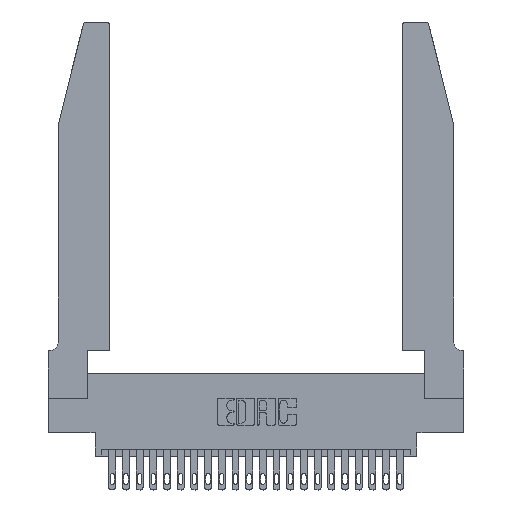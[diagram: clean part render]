
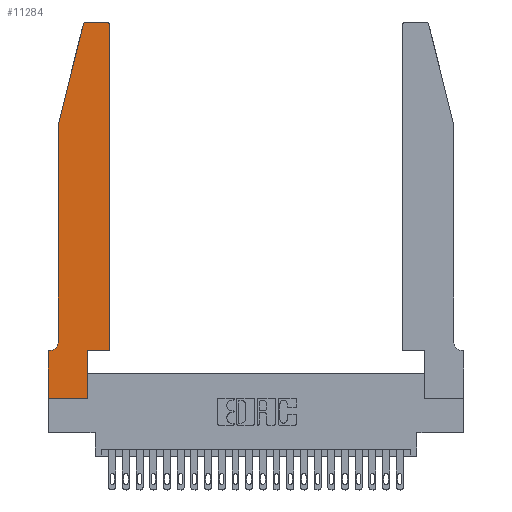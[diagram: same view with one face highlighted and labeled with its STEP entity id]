
A CAD part, top view. The second image highlights one B-rep face of the part: STEP entity #11284.
In plain terms, the highlighted planar face has unit normal (0, 0, 1).
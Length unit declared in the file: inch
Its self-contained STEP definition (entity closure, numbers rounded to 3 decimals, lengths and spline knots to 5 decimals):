
#243 = CARTESIAN_POINT ( 'NONE',  ( 0., 0., 0.37 ) ) ;
#632 = CARTESIAN_POINT ( 'NONE',  ( 0.284, 2.72, 0.37 ) ) ;
#1090 = DIRECTION ( 'NONE',  ( 0., 1., 0. ) ) ;
#1114 = AXIS2_PLACEMENT_3D ( 'NONE', #22229, #24005, #10795 ) ;
#1172 = ORIENTED_EDGE ( 'NONE', *, *, #23005, .T. ) ;
#1289 = CARTESIAN_POINT ( 'NONE',  ( 0.4505, 0.35, 0.37 ) ) ;
#1506 = CARTESIAN_POINT ( 'NONE',  ( 0.0755, 2., 0.37 ) ) ;
#1558 = EDGE_CURVE ( 'NONE', #6737, #5088, #21562, .T. ) ;
#1679 = VECTOR ( 'NONE', #21174, 39.37008 ) ;
#2625 = EDGE_CURVE ( 'NONE', #9777, #20598, #21193, .T. ) ;
#3010 = CARTESIAN_POINT ( 'NONE',  ( 0.4505, 0.35, 0.37 ) ) ;
#3607 = VERTEX_POINT ( 'NONE', #9351 ) ;
#4020 = VECTOR ( 'NONE', #17602, 39.37008 ) ;
#4476 = VERTEX_POINT ( 'NONE', #9982 ) ;
#4489 = ORIENTED_EDGE ( 'NONE', *, *, #22516, .T. ) ;
#4597 = EDGE_CURVE ( 'NONE', #6879, #9777, #5947, .T. ) ;
#5088 = VERTEX_POINT ( 'NONE', #24771 ) ;
#5301 = VECTOR ( 'NONE', #10873, 39.37008 ) ;
#5439 = VERTEX_POINT ( 'NONE', #10442 ) ;
#5543 = CARTESIAN_POINT ( 'NONE',  ( 0.2865, 0.35, 0.37 ) ) ;
#5947 = LINE ( 'NONE', #21570, #7403 ) ;
#6316 = CARTESIAN_POINT ( 'NONE',  ( 0., 0.35, 0.37 ) ) ;
#6472 = EDGE_LOOP ( 'NONE', ( #16939, #22585, #20872, #4489, #13615, #19061, #1172, #21306, #22916, #13959, #22687, #8052 ) ) ;
#6713 = LINE ( 'NONE', #8328, #7008 ) ;
#6737 = VERTEX_POINT ( 'NONE', #15553 ) ;
#6823 = VECTOR ( 'NONE', #16978, 39.37008 ) ;
#6879 = VERTEX_POINT ( 'NONE', #12028 ) ;
#7008 = VECTOR ( 'NONE', #12144, 39.37008 ) ;
#7403 = VECTOR ( 'NONE', #21819, 39.37008 ) ;
#7823 = AXIS2_PLACEMENT_3D ( 'NONE', #632, #19560, #13900 ) ;
#7963 = LINE ( 'NONE', #13411, #1679 ) ;
#7984 = DIRECTION ( 'NONE',  ( 1., 0., 0. ) ) ;
#8018 = EDGE_CURVE ( 'NONE', #11423, #15304, #6713, .T. ) ;
#8052 = ORIENTED_EDGE ( 'NONE', *, *, #22491, .T. ) ;
#8270 = CIRCLE ( 'NONE', #1114, 0.03 ) ;
#8328 = CARTESIAN_POINT ( 'NONE',  ( 0.0755, 2., 0.37 ) ) ;
#8665 = VECTOR ( 'NONE', #1090, 39.37008 ) ;
#9351 = CARTESIAN_POINT ( 'NONE',  ( 0.284, 2.75, 0.37 ) ) ;
#9777 = VERTEX_POINT ( 'NONE', #1289 ) ;
#9982 = CARTESIAN_POINT ( 'NONE',  ( 0.4205, 2.75, 0.37 ) ) ;
#10442 = CARTESIAN_POINT ( 'NONE',  ( 0., 0., 0.37 ) ) ;
#10482 = CARTESIAN_POINT ( 'NONE',  ( 0.25487, 2.72718, 0.37 ) ) ;
#10795 = DIRECTION ( 'NONE',  ( 1., 0., 0. ) ) ;
#10873 = DIRECTION ( 'NONE',  ( 0., -1., 0. ) ) ;
#11075 = VECTOR ( 'NONE', #13660, 39.37008 ) ;
#11284 = ADVANCED_FACE ( 'NONE', ( #23284 ), #14061, .T. ) ;
#11423 = VERTEX_POINT ( 'NONE', #10482 ) ;
#11638 = EDGE_CURVE ( 'NONE', #21131, #6879, #20835, .T. ) ;
#12028 = CARTESIAN_POINT ( 'NONE',  ( 0.2865, 0.35, 0.37 ) ) ;
#12144 = DIRECTION ( 'NONE',  ( -0.239, -0.971, 0. ) ) ;
#12452 = LINE ( 'NONE', #12698, #5301 ) ;
#12698 = CARTESIAN_POINT ( 'NONE',  ( 0.0755, 2., 0.37 ) ) ;
#13148 = VERTEX_POINT ( 'NONE', #19773 ) ;
#13311 = DIRECTION ( 'NONE',  ( 0., 0., -1. ) ) ;
#13411 = CARTESIAN_POINT ( 'NONE',  ( 0.0755, 0.35, 0.37 ) ) ;
#13615 = ORIENTED_EDGE ( 'NONE', *, *, #1558, .T. ) ;
#13660 = DIRECTION ( 'NONE',  ( 1., 0., 0. ) ) ;
#13900 = DIRECTION ( 'NONE',  ( 1., 0., 0. ) ) ;
#13959 = ORIENTED_EDGE ( 'NONE', *, *, #4597, .T. ) ;
#14061 = PLANE ( 'NONE',  #16128 ) ;
#15177 = DIRECTION ( 'NONE',  ( -1., 0., 0. ) ) ;
#15304 = VERTEX_POINT ( 'NONE', #1506 ) ;
#15553 = CARTESIAN_POINT ( 'NONE',  ( 0.0755, 0.42, 0.37 ) ) ;
#15942 = EDGE_CURVE ( 'NONE', #5439, #21131, #20012, .T. ) ;
#16128 = AXIS2_PLACEMENT_3D ( 'NONE', #6316, #19468, #7984 ) ;
#16269 = DIRECTION ( 'NONE',  ( 0., -1., 0. ) ) ;
#16939 = ORIENTED_EDGE ( 'NONE', *, *, #24687, .T. ) ;
#16978 = DIRECTION ( 'NONE',  ( 0., 1., 0. ) ) ;
#17602 = DIRECTION ( 'NONE',  ( -1., 0., 0. ) ) ;
#18172 = CARTESIAN_POINT ( 'NONE',  ( 0., 0., 0.37 ) ) ;
#18385 = LINE ( 'NONE', #18172, #19258 ) ;
#18426 = EDGE_CURVE ( 'NONE', #5088, #13148, #7963, .T. ) ;
#18915 = LINE ( 'NONE', #19741, #4020 ) ;
#19061 = ORIENTED_EDGE ( 'NONE', *, *, #18426, .T. ) ;
#19073 = CARTESIAN_POINT ( 'NONE',  ( 0.0055, 0.42, 0.37 ) ) ;
#19258 = VECTOR ( 'NONE', #16269, 39.37008 ) ;
#19468 = DIRECTION ( 'NONE',  ( 0., 0., 1. ) ) ;
#19560 = DIRECTION ( 'NONE',  ( 0., 0., 1. ) ) ;
#19741 = CARTESIAN_POINT ( 'NONE',  ( 0.2605, 2.75, 0.37 ) ) ;
#19773 = CARTESIAN_POINT ( 'NONE',  ( 0., 0.35, 0.37 ) ) ;
#20012 = LINE ( 'NONE', #243, #11075 ) ;
#20598 = VERTEX_POINT ( 'NONE', #24131 ) ;
#20740 = CIRCLE ( 'NONE', #7823, 0.03 ) ;
#20835 = LINE ( 'NONE', #5543, #6823 ) ;
#20872 = ORIENTED_EDGE ( 'NONE', *, *, #8018, .T. ) ;
#21131 = VERTEX_POINT ( 'NONE', #23972 ) ;
#21174 = DIRECTION ( 'NONE',  ( -1., 0., 0. ) ) ;
#21193 = LINE ( 'NONE', #3010, #8665 ) ;
#21306 = ORIENTED_EDGE ( 'NONE', *, *, #15942, .T. ) ;
#21562 = CIRCLE ( 'NONE', #24010, 0.07 ) ;
#21570 = CARTESIAN_POINT ( 'NONE',  ( 0.4505, 0.35, 0.37 ) ) ;
#21819 = DIRECTION ( 'NONE',  ( 1., 0., 0. ) ) ;
#22229 = CARTESIAN_POINT ( 'NONE',  ( 0.4205, 2.72, 0.37 ) ) ;
#22491 = EDGE_CURVE ( 'NONE', #20598, #4476, #8270, .T. ) ;
#22516 = EDGE_CURVE ( 'NONE', #15304, #6737, #12452, .T. ) ;
#22585 = ORIENTED_EDGE ( 'NONE', *, *, #23507, .T. ) ;
#22687 = ORIENTED_EDGE ( 'NONE', *, *, #2625, .T. ) ;
#22916 = ORIENTED_EDGE ( 'NONE', *, *, #11638, .T. ) ;
#23005 = EDGE_CURVE ( 'NONE', #13148, #5439, #18385, .T. ) ;
#23284 = FACE_OUTER_BOUND ( 'NONE', #6472, .T. ) ;
#23507 = EDGE_CURVE ( 'NONE', #3607, #11423, #20740, .T. ) ;
#23972 = CARTESIAN_POINT ( 'NONE',  ( 0.2865, 0., 0.37 ) ) ;
#24005 = DIRECTION ( 'NONE',  ( 0., 0., 1. ) ) ;
#24010 = AXIS2_PLACEMENT_3D ( 'NONE', #19073, #13311, #15177 ) ;
#24131 = CARTESIAN_POINT ( 'NONE',  ( 0.4505, 2.72, 0.37 ) ) ;
#24687 = EDGE_CURVE ( 'NONE', #4476, #3607, #18915, .T. ) ;
#24771 = CARTESIAN_POINT ( 'NONE',  ( 0.0055, 0.35, 0.37 ) ) ;
